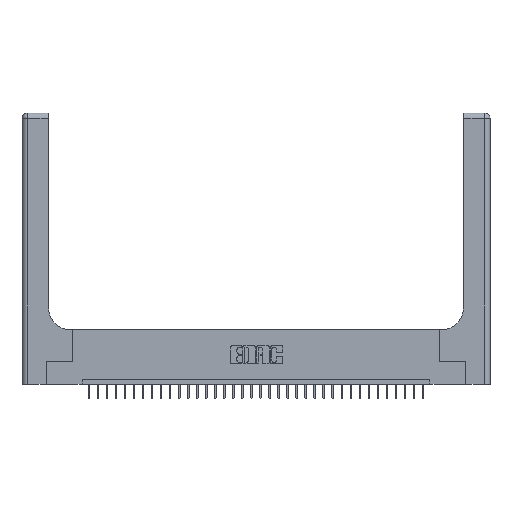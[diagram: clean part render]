
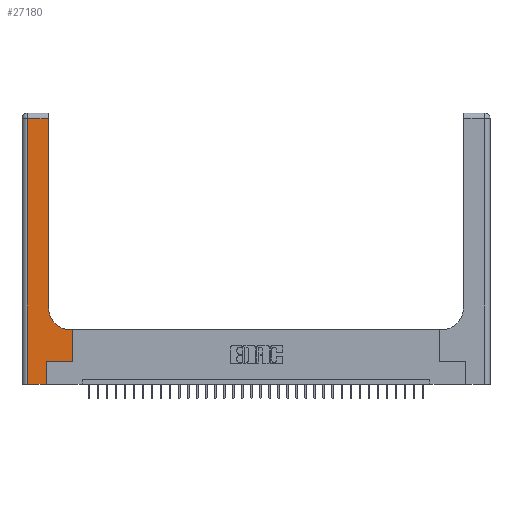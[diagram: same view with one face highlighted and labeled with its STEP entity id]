
A CAD part, top view. The second image highlights one B-rep face of the part: STEP entity #27180.
In plain terms, the highlighted planar face has unit normal (0, 0, 1).
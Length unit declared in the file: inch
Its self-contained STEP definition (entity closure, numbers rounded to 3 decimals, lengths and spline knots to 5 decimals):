
#1083 = AXIS2_PLACEMENT_3D ( 'NONE', #8752, #3309, #30051 ) ;
#1329 = CARTESIAN_POINT ( 'NONE',  ( 0.2915, 0.85, 0.37 ) ) ;
#2749 = CARTESIAN_POINT ( 'NONE',  ( 0.269, 0., 0.37 ) ) ;
#3309 = DIRECTION ( 'NONE',  ( 0., 0., -1. ) ) ;
#3396 = VERTEX_POINT ( 'NONE', #26495 ) ;
#4316 = CARTESIAN_POINT ( 'NONE',  ( 0.269, 0., 0.37 ) ) ;
#4366 = VECTOR ( 'NONE', #18446, 39.37008 ) ;
#4977 = DIRECTION ( 'NONE',  ( 0., -1., 0. ) ) ;
#7437 = DIRECTION ( 'NONE',  ( 1., 0., 0. ) ) ;
#7450 = CARTESIAN_POINT ( 'NONE',  ( 0.5585, 0.25, 0.37 ) ) ;
#7757 = CIRCLE ( 'NONE', #1083, 0.25 ) ;
#7796 = CARTESIAN_POINT ( 'NONE',  ( 0.2915, 2.94, 0.37 ) ) ;
#7819 = VECTOR ( 'NONE', #9734, 39.37008 ) ;
#7933 = VERTEX_POINT ( 'NONE', #4316 ) ;
#8318 = LINE ( 'NONE', #28238, #16606 ) ;
#8402 = VERTEX_POINT ( 'NONE', #30946 ) ;
#8752 = CARTESIAN_POINT ( 'NONE',  ( 0.5415, 0.85, 0.37 ) ) ;
#8913 = EDGE_CURVE ( 'NONE', #14838, #9143, #21574, .T. ) ;
#9074 = EDGE_CURVE ( 'NONE', #9143, #31604, #18638, .T. ) ;
#9143 = VERTEX_POINT ( 'NONE', #15573 ) ;
#9151 = ORIENTED_EDGE ( 'NONE', *, *, #15490, .T. ) ;
#9734 = DIRECTION ( 'NONE',  ( -1., 0., 0. ) ) ;
#10106 = ORIENTED_EDGE ( 'NONE', *, *, #11603, .T. ) ;
#10574 = DIRECTION ( 'NONE',  ( 1., 0., 0. ) ) ;
#10811 = EDGE_CURVE ( 'NONE', #8402, #3396, #15149, .T. ) ;
#10932 = ORIENTED_EDGE ( 'NONE', *, *, #10811, .T. ) ;
#11140 = DIRECTION ( 'NONE',  ( 0., 0., -1. ) ) ;
#11272 = VERTEX_POINT ( 'NONE', #20805 ) ;
#11603 = EDGE_CURVE ( 'NONE', #34107, #14838, #21465, .T. ) ;
#11618 = AXIS2_PLACEMENT_3D ( 'NONE', #24418, #11140, #32185 ) ;
#12286 = CARTESIAN_POINT ( 'NONE',  ( 0., 2.94, 0.37 ) ) ;
#12647 = DIRECTION ( 'NONE',  ( 0., 1., 0. ) ) ;
#13614 = CARTESIAN_POINT ( 'NONE',  ( 0.2915, 3., 0.37 ) ) ;
#14415 = CARTESIAN_POINT ( 'NONE',  ( 0.06, 0., 0.37 ) ) ;
#14838 = VERTEX_POINT ( 'NONE', #7796 ) ;
#15034 = EDGE_CURVE ( 'NONE', #11272, #8402, #15402, .T. ) ;
#15149 = LINE ( 'NONE', #33907, #34292 ) ;
#15343 = EDGE_LOOP ( 'NONE', ( #10106, #24216, #31766, #19335, #28974, #9151, #21551, #10932, #17852 ) ) ;
#15402 = LINE ( 'NONE', #7450, #24593 ) ;
#15490 = EDGE_CURVE ( 'NONE', #32657, #11272, #8318, .T. ) ;
#15573 = CARTESIAN_POINT ( 'NONE',  ( 0.06, 2.94, 0.37 ) ) ;
#16606 = VECTOR ( 'NONE', #7437, 39.37008 ) ;
#17852 = ORIENTED_EDGE ( 'NONE', *, *, #21590, .T. ) ;
#18166 = LINE ( 'NONE', #20953, #31490 ) ;
#18446 = DIRECTION ( 'NONE',  ( 0., 1., 0. ) ) ;
#18572 = FACE_OUTER_BOUND ( 'NONE', #15343, .T. ) ;
#18638 = LINE ( 'NONE', #22198, #22372 ) ;
#19335 = ORIENTED_EDGE ( 'NONE', *, *, #27063, .T. ) ;
#20805 = CARTESIAN_POINT ( 'NONE',  ( 0.5585, 0.25, 0.37 ) ) ;
#20953 = CARTESIAN_POINT ( 'NONE',  ( 0., 0., 0.37 ) ) ;
#21353 = CARTESIAN_POINT ( 'NONE',  ( 0.269, 0.25, 0.37 ) ) ;
#21465 = LINE ( 'NONE', #13614, #27670 ) ;
#21551 = ORIENTED_EDGE ( 'NONE', *, *, #15034, .T. ) ;
#21574 = LINE ( 'NONE', #12286, #7819 ) ;
#21590 = EDGE_CURVE ( 'NONE', #3396, #34107, #7757, .T. ) ;
#21740 = PLANE ( 'NONE',  #11618 ) ;
#21852 = LINE ( 'NONE', #2749, #4366 ) ;
#22198 = CARTESIAN_POINT ( 'NONE',  ( 0.06, 3., 0.37 ) ) ;
#22372 = VECTOR ( 'NONE', #4977, 39.37008 ) ;
#22805 = EDGE_CURVE ( 'NONE', #7933, #32657, #21852, .T. ) ;
#24216 = ORIENTED_EDGE ( 'NONE', *, *, #8913, .T. ) ;
#24418 = CARTESIAN_POINT ( 'NONE',  ( 0., 3., 0.37 ) ) ;
#24593 = VECTOR ( 'NONE', #12647, 39.37008 ) ;
#26088 = DIRECTION ( 'NONE',  ( -1., 0., 0. ) ) ;
#26495 = CARTESIAN_POINT ( 'NONE',  ( 0.5415, 0.6, 0.37 ) ) ;
#27063 = EDGE_CURVE ( 'NONE', #31604, #7933, #18166, .T. ) ;
#27180 = ADVANCED_FACE ( 'NONE', ( #18572 ), #21740, .F. ) ;
#27441 = DIRECTION ( 'NONE',  ( 0., 1., 0. ) ) ;
#27670 = VECTOR ( 'NONE', #27441, 39.37008 ) ;
#28238 = CARTESIAN_POINT ( 'NONE',  ( 0.269, 0.25, 0.37 ) ) ;
#28974 = ORIENTED_EDGE ( 'NONE', *, *, #22805, .T. ) ;
#30051 = DIRECTION ( 'NONE',  ( 1., 0., 0. ) ) ;
#30946 = CARTESIAN_POINT ( 'NONE',  ( 0.5585, 0.6, 0.37 ) ) ;
#31490 = VECTOR ( 'NONE', #10574, 39.37008 ) ;
#31604 = VERTEX_POINT ( 'NONE', #14415 ) ;
#31766 = ORIENTED_EDGE ( 'NONE', *, *, #9074, .T. ) ;
#32185 = DIRECTION ( 'NONE',  ( -1., 0., 0. ) ) ;
#32657 = VERTEX_POINT ( 'NONE', #21353 ) ;
#33907 = CARTESIAN_POINT ( 'NONE',  ( 0.2915, 0.6, 0.37 ) ) ;
#34107 = VERTEX_POINT ( 'NONE', #1329 ) ;
#34292 = VECTOR ( 'NONE', #26088, 39.37008 ) ;
